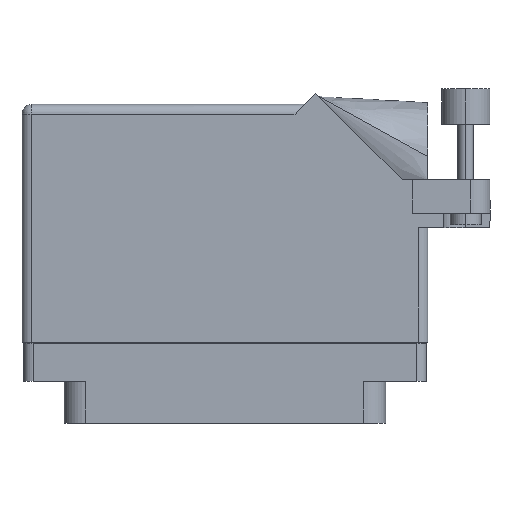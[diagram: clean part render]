
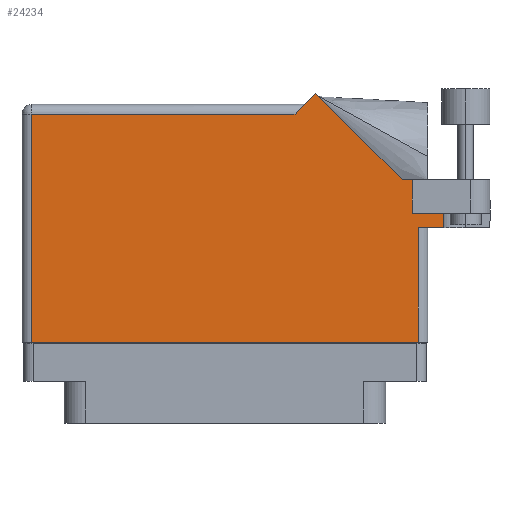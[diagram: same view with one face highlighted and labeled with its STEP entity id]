
A CAD part, front view. The second image highlights one B-rep face of the part: STEP entity #24234.
In plain terms, the highlighted face is planar.
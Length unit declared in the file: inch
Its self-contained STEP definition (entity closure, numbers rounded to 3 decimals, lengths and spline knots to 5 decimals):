
#2886 = CARTESIAN_POINT ( 'NONE',  ( 1.14042, 0.944, 0.455 ) ) ;
#3422 = EDGE_CURVE ( 'NONE', #44807, #32247, #13653, .T. ) ;
#4180 = LINE ( 'NONE', #16991, #17017 ) ;
#4662 = EDGE_CURVE ( 'NONE', #10222, #31058, #39205, .T. ) ;
#5094 = LINE ( 'NONE', #5711, #43480 ) ;
#5711 = CARTESIAN_POINT ( 'NONE',  ( 1.14042, 0.944, 0.455 ) ) ;
#6582 = VERTEX_POINT ( 'NONE', #2886 ) ;
#6785 = EDGE_CURVE ( 'NONE', #14452, #15819, #14326, .T. ) ;
#7227 = DIRECTION ( 'NONE',  ( -1., 0., 0. ) ) ;
#7304 = CARTESIAN_POINT ( 'NONE',  ( 1.206, 0.731, 0.455 ) ) ;
#7666 = LINE ( 'NONE', #11750, #38543 ) ;
#8402 = ORIENTED_EDGE ( 'NONE', *, *, #42994, .F. ) ;
#8568 = CARTESIAN_POINT ( 'NONE',  ( 0.513, 1.43, 0.455 ) ) ;
#10222 = VERTEX_POINT ( 'NONE', #31018 ) ;
#10594 = DIRECTION ( 'NONE',  ( 0., -1., 0. ) ) ;
#10997 = DIRECTION ( 'NONE',  ( 1., 0., 0. ) ) ;
#11300 = CARTESIAN_POINT ( 'NONE',  ( 1.306, 0.637, 0.455 ) ) ;
#11750 = CARTESIAN_POINT ( 'NONE',  ( 1.206, 0.731, 0.455 ) ) ;
#12108 = CARTESIAN_POINT ( 'NONE',  ( 1.4075, 1.06177, 0.455 ) ) ;
#12521 = CARTESIAN_POINT ( 'NONE',  ( 1.4075, 0.637, 0.455 ) ) ;
#12756 = ORIENTED_EDGE ( 'NONE', *, *, #4662, .T. ) ;
#13183 = ORIENTED_EDGE ( 'NONE', *, *, #14017, .T. ) ;
#13511 = LINE ( 'NONE', #12108, #22184 ) ;
#13595 = PLANE ( 'NONE',  #28157 ) ;
#13653 = LINE ( 'NONE', #28334, #20634 ) ;
#14017 = EDGE_CURVE ( 'NONE', #31058, #31422, #32771, .T. ) ;
#14120 = VECTOR ( 'NONE', #10594, 39.37008 ) ;
#14326 = LINE ( 'NONE', #8568, #47495 ) ;
#14452 = VERTEX_POINT ( 'NONE', #32034 ) ;
#14637 = ORIENTED_EDGE ( 'NONE', *, *, #6785, .T. ) ;
#15819 = VERTEX_POINT ( 'NONE', #26058 ) ;
#16941 = DIRECTION ( 'NONE',  ( 0., 1., 0. ) ) ;
#16991 = CARTESIAN_POINT ( 'NONE',  ( -1.306, 1.368, 0.455 ) ) ;
#17017 = VECTOR ( 'NONE', #36848, 39.37008 ) ;
#17321 = DIRECTION ( 'NONE',  ( -1., 0., 0. ) ) ;
#17839 = LINE ( 'NONE', #22449, #46378 ) ;
#18691 = CARTESIAN_POINT ( 'NONE',  ( -1.244, -0.1, 0.455 ) ) ;
#20634 = VECTOR ( 'NONE', #16941, 39.37008 ) ;
#21815 = DIRECTION ( 'NONE',  ( 1., 0., 0. ) ) ;
#21928 = ORIENTED_EDGE ( 'NONE', *, *, #42849, .T. ) ;
#22184 = VECTOR ( 'NONE', #41572, 39.37008 ) ;
#22449 = CARTESIAN_POINT ( 'NONE',  ( 1.706, 0.944, 0.455 ) ) ;
#22510 = VERTEX_POINT ( 'NONE', #12521 ) ;
#22806 = ORIENTED_EDGE ( 'NONE', *, *, #39667, .T. ) ;
#22915 = DIRECTION ( 'NONE',  ( 1., 0., 0. ) ) ;
#23205 = FACE_OUTER_BOUND ( 'NONE', #44097, .T. ) ;
#24234 = ADVANCED_FACE ( 'NONE', ( #23205 ), #13595, .F. ) ;
#24281 = CARTESIAN_POINT ( 'NONE',  ( -1.306, 1.43, 0.455 ) ) ;
#24644 = VECTOR ( 'NONE', #28361, 39.37008 ) ;
#26058 = CARTESIAN_POINT ( 'NONE',  ( 0.451, 1.368, 0.455 ) ) ;
#26882 = VECTOR ( 'NONE', #10997, 39.37008 ) ;
#26985 = VERTEX_POINT ( 'NONE', #39848 ) ;
#27835 = ORIENTED_EDGE ( 'NONE', *, *, #29131, .T. ) ;
#27891 = CARTESIAN_POINT ( 'NONE',  ( 1.244, 0.637, 0.455 ) ) ;
#28090 = DIRECTION ( 'NONE',  ( 0., 0., -1. ) ) ;
#28120 = DIRECTION ( 'NONE',  ( -0.707, 0.707, 0. ) ) ;
#28157 = AXIS2_PLACEMENT_3D ( 'NONE', #24281, #28090, #17321 ) ;
#28334 = CARTESIAN_POINT ( 'NONE',  ( 1.206, 0.731, 0.455 ) ) ;
#28361 = DIRECTION ( 'NONE',  ( 0., 1., 0. ) ) ;
#28822 = ORIENTED_EDGE ( 'NONE', *, *, #3422, .T. ) ;
#29131 = EDGE_CURVE ( 'NONE', #32247, #6582, #17839, .T. ) ;
#29942 = CARTESIAN_POINT ( 'NONE',  ( -1.306, -0.1, 0.455 ) ) ;
#30106 = CARTESIAN_POINT ( 'NONE',  ( 1.206, 0.944, 0.455 ) ) ;
#31018 = CARTESIAN_POINT ( 'NONE',  ( -1.244, 1.368, 0.455 ) ) ;
#31058 = VERTEX_POINT ( 'NONE', #47346 ) ;
#31422 = VERTEX_POINT ( 'NONE', #41994 ) ;
#32034 = CARTESIAN_POINT ( 'NONE',  ( 0.58371, 1.50071, 0.455 ) ) ;
#32247 = VERTEX_POINT ( 'NONE', #30106 ) ;
#32771 = LINE ( 'NONE', #29942, #40391 ) ;
#34773 = EDGE_CURVE ( 'NONE', #15819, #10222, #4180, .T. ) ;
#36566 = ORIENTED_EDGE ( 'NONE', *, *, #41174, .F. ) ;
#36848 = DIRECTION ( 'NONE',  ( -1., 0., 0. ) ) ;
#37512 = CARTESIAN_POINT ( 'NONE',  ( 1.244, 0.637, 0.455 ) ) ;
#38543 = VECTOR ( 'NONE', #22915, 39.37008 ) ;
#38547 = ORIENTED_EDGE ( 'NONE', *, *, #46407, .T. ) ;
#39205 = LINE ( 'NONE', #18691, #14120 ) ;
#39667 = EDGE_CURVE ( 'NONE', #31422, #47321, #43869, .T. ) ;
#39848 = CARTESIAN_POINT ( 'NONE',  ( 1.4075, 0.731, 0.455 ) ) ;
#40391 = VECTOR ( 'NONE', #21815, 39.37008 ) ;
#41174 = EDGE_CURVE ( 'NONE', #44807, #26985, #7666, .T. ) ;
#41572 = DIRECTION ( 'NONE',  ( 0., -1., 0. ) ) ;
#41994 = CARTESIAN_POINT ( 'NONE',  ( 1.244, -0.1, 0.455 ) ) ;
#42020 = LINE ( 'NONE', #11300, #26882 ) ;
#42849 = EDGE_CURVE ( 'NONE', #47321, #22510, #42020, .T. ) ;
#42909 = DIRECTION ( 'NONE',  ( -0.707, -0.707, 0. ) ) ;
#42994 = EDGE_CURVE ( 'NONE', #26985, #22510, #13511, .T. ) ;
#43480 = VECTOR ( 'NONE', #28120, 39.37008 ) ;
#43869 = LINE ( 'NONE', #27891, #24644 ) ;
#44097 = EDGE_LOOP ( 'NONE', ( #13183, #22806, #21928, #8402, #36566, #28822, #27835, #38547, #14637, #47711, #12756 ) ) ;
#44807 = VERTEX_POINT ( 'NONE', #7304 ) ;
#46378 = VECTOR ( 'NONE', #7227, 39.37008 ) ;
#46407 = EDGE_CURVE ( 'NONE', #6582, #14452, #5094, .T. ) ;
#47321 = VERTEX_POINT ( 'NONE', #37512 ) ;
#47346 = CARTESIAN_POINT ( 'NONE',  ( -1.244, -0.1, 0.455 ) ) ;
#47495 = VECTOR ( 'NONE', #42909, 39.37008 ) ;
#47711 = ORIENTED_EDGE ( 'NONE', *, *, #34773, .T. ) ;
